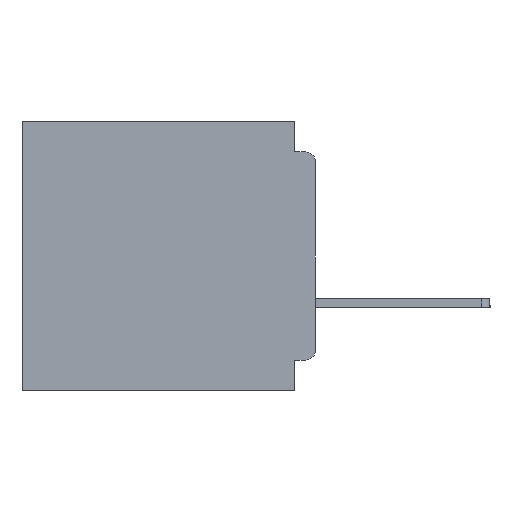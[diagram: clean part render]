
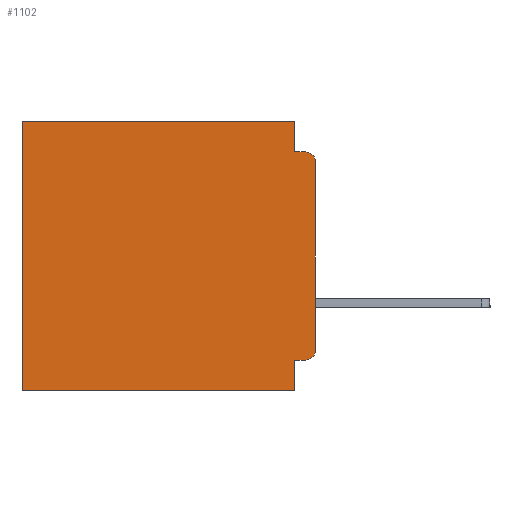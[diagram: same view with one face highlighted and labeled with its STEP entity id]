
A CAD part, left-side view. The second image highlights one B-rep face of the part: STEP entity #1102.
In plain terms, the highlighted planar face has unit normal (-1, 0, 0).
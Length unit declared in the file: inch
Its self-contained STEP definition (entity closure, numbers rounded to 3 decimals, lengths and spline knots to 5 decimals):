
#610 = CARTESIAN_POINT ( 'NONE',  ( 0.3, 0.437, -0.4 ) ) ;
#1047 = DIRECTION ( 'NONE',  ( 0., 0., -1. ) ) ;
#1063 = EDGE_CURVE ( 'NONE', #3150, #40038, #52916, .T. ) ;
#1102 = ADVANCED_FACE ( 'NONE', ( #39441 ), #8871, .F. ) ;
#1307 = CARTESIAN_POINT ( 'NONE',  ( 0.3, 0.031, 0. ) ) ;
#1870 = VECTOR ( 'NONE', #16894, 39.37008 ) ;
#2061 = EDGE_CURVE ( 'NONE', #35365, #28971, #36208, .T. ) ;
#3041 = AXIS2_PLACEMENT_3D ( 'NONE', #30626, #5924, #34715 ) ;
#3150 = VERTEX_POINT ( 'NONE', #31823 ) ;
#3378 = CARTESIAN_POINT ( 'NONE',  ( 0.3, 0.031, -0.355 ) ) ;
#3846 = VECTOR ( 'NONE', #20789, 39.37008 ) ;
#4643 = CARTESIAN_POINT ( 'NONE',  ( 0.3, 0., -0.045 ) ) ;
#5272 = VECTOR ( 'NONE', #29360, 39.37008 ) ;
#5924 = DIRECTION ( 'NONE',  ( -1., 0., 0. ) ) ;
#6433 = LINE ( 'NONE', #41246, #3846 ) ;
#6959 = VERTEX_POINT ( 'NONE', #25955 ) ;
#7569 = EDGE_CURVE ( 'NONE', #3150, #6959, #26277, .T. ) ;
#8660 = ORIENTED_EDGE ( 'NONE', *, *, #46248, .T. ) ;
#8871 = PLANE ( 'NONE',  #51814 ) ;
#9040 = CIRCLE ( 'NONE', #3041, 0.015 ) ;
#9572 = ORIENTED_EDGE ( 'NONE', *, *, #32262, .F. ) ;
#12952 = VECTOR ( 'NONE', #17056, 39.37008 ) ;
#14262 = LINE ( 'NONE', #610, #12952 ) ;
#15152 = CARTESIAN_POINT ( 'NONE',  ( 0.3, 0.437, 0. ) ) ;
#15314 = VECTOR ( 'NONE', #21934, 39.37008 ) ;
#16266 = LINE ( 'NONE', #4643, #5272 ) ;
#16894 = DIRECTION ( 'NONE',  ( 0., 0., -1. ) ) ;
#17056 = DIRECTION ( 'NONE',  ( 0., 0., -1. ) ) ;
#17209 = CARTESIAN_POINT ( 'NONE',  ( 0.3, 0., -0.355 ) ) ;
#17351 = AXIS2_PLACEMENT_3D ( 'NONE', #47385, #22800, #51494 ) ;
#19828 = CARTESIAN_POINT ( 'NONE',  ( 0.3, 0.015, -0.355 ) ) ;
#20005 = CARTESIAN_POINT ( 'NONE',  ( 0.3, 0.031, -0.4 ) ) ;
#20697 = EDGE_CURVE ( 'NONE', #37689, #28971, #9040, .T. ) ;
#20789 = DIRECTION ( 'NONE',  ( 0., 1., 0. ) ) ;
#21307 = ORIENTED_EDGE ( 'NONE', *, *, #1063, .T. ) ;
#21934 = DIRECTION ( 'NONE',  ( 0., 0., -1. ) ) ;
#22800 = DIRECTION ( 'NONE',  ( -1., 0., 0. ) ) ;
#25955 = CARTESIAN_POINT ( 'NONE',  ( 0.3, 0.031, -0.045 ) ) ;
#26199 = CARTESIAN_POINT ( 'NONE',  ( 0.3, 0.015, -0.045 ) ) ;
#26277 = LINE ( 'NONE', #1307, #15314 ) ;
#28971 = VERTEX_POINT ( 'NONE', #47259 ) ;
#29360 = DIRECTION ( 'NONE',  ( 0., -1., 0. ) ) ;
#29813 = CARTESIAN_POINT ( 'NONE',  ( 0.3, 0., -0.4 ) ) ;
#30626 = CARTESIAN_POINT ( 'NONE',  ( 0.3, 0.015, -0.34 ) ) ;
#31122 = VECTOR ( 'NONE', #52770, 39.37008 ) ;
#31194 = VECTOR ( 'NONE', #41853, 39.37008 ) ;
#31314 = VERTEX_POINT ( 'NONE', #26199 ) ;
#31823 = CARTESIAN_POINT ( 'NONE',  ( 0.3, 0.031, 0. ) ) ;
#32262 = EDGE_CURVE ( 'NONE', #37689, #34897, #40805, .T. ) ;
#33429 = CARTESIAN_POINT ( 'NONE',  ( 0.3, 0.031, -0.4 ) ) ;
#33524 = ORIENTED_EDGE ( 'NONE', *, *, #7569, .F. ) ;
#33843 = DIRECTION ( 'NONE',  ( 0., 0., -1. ) ) ;
#34715 = DIRECTION ( 'NONE',  ( 0., 0., -1. ) ) ;
#34741 = LINE ( 'NONE', #33429, #1870 ) ;
#34897 = VERTEX_POINT ( 'NONE', #3378 ) ;
#35365 = VERTEX_POINT ( 'NONE', #47432 ) ;
#36200 = DIRECTION ( 'NONE',  ( 1., 0., 0. ) ) ;
#36208 = LINE ( 'NONE', #42643, #45879 ) ;
#36553 = VERTEX_POINT ( 'NONE', #47856 ) ;
#36697 = VERTEX_POINT ( 'NONE', #20005 ) ;
#37245 = EDGE_CURVE ( 'NONE', #36697, #36553, #6433, .T. ) ;
#37689 = VERTEX_POINT ( 'NONE', #19828 ) ;
#38895 = ORIENTED_EDGE ( 'NONE', *, *, #2061, .F. ) ;
#39441 = FACE_OUTER_BOUND ( 'NONE', #40668, .T. ) ;
#39531 = CIRCLE ( 'NONE', #17351, 0.015 ) ;
#39659 = ORIENTED_EDGE ( 'NONE', *, *, #50628, .T. ) ;
#40038 = VERTEX_POINT ( 'NONE', #15152 ) ;
#40317 = EDGE_CURVE ( 'NONE', #6959, #31314, #16266, .T. ) ;
#40668 = EDGE_LOOP ( 'NONE', ( #38895, #8660, #48822, #33524, #21307, #39659, #41420, #44253, #9572, #47526 ) ) ;
#40805 = LINE ( 'NONE', #17209, #31194 ) ;
#41246 = CARTESIAN_POINT ( 'NONE',  ( 0.3, 0., -0.4 ) ) ;
#41420 = ORIENTED_EDGE ( 'NONE', *, *, #37245, .F. ) ;
#41853 = DIRECTION ( 'NONE',  ( 0., 1., 0. ) ) ;
#42643 = CARTESIAN_POINT ( 'NONE',  ( 0.3, 0., -0.4 ) ) ;
#44253 = ORIENTED_EDGE ( 'NONE', *, *, #48695, .F. ) ;
#45879 = VECTOR ( 'NONE', #1047, 39.37008 ) ;
#46248 = EDGE_CURVE ( 'NONE', #35365, #31314, #39531, .T. ) ;
#47259 = CARTESIAN_POINT ( 'NONE',  ( 0.3, 0., -0.34 ) ) ;
#47385 = CARTESIAN_POINT ( 'NONE',  ( 0.3, 0.015, -0.06 ) ) ;
#47432 = CARTESIAN_POINT ( 'NONE',  ( 0.3, 0., -0.06 ) ) ;
#47526 = ORIENTED_EDGE ( 'NONE', *, *, #20697, .T. ) ;
#47856 = CARTESIAN_POINT ( 'NONE',  ( 0.3, 0.437, -0.4 ) ) ;
#48695 = EDGE_CURVE ( 'NONE', #34897, #36697, #34741, .T. ) ;
#48822 = ORIENTED_EDGE ( 'NONE', *, *, #40317, .F. ) ;
#50628 = EDGE_CURVE ( 'NONE', #40038, #36553, #14262, .T. ) ;
#51494 = DIRECTION ( 'NONE',  ( 0., 0., -1. ) ) ;
#51814 = AXIS2_PLACEMENT_3D ( 'NONE', #29813, #36200, #33843 ) ;
#52590 = CARTESIAN_POINT ( 'NONE',  ( 0.3, 0., 0. ) ) ;
#52770 = DIRECTION ( 'NONE',  ( 0., 1., 0. ) ) ;
#52916 = LINE ( 'NONE', #52590, #31122 ) ;
